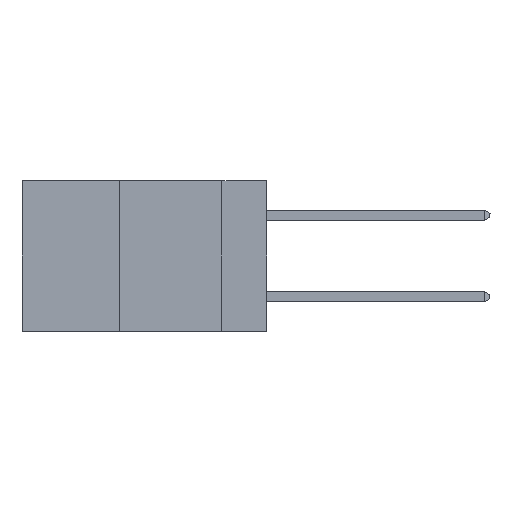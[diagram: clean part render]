
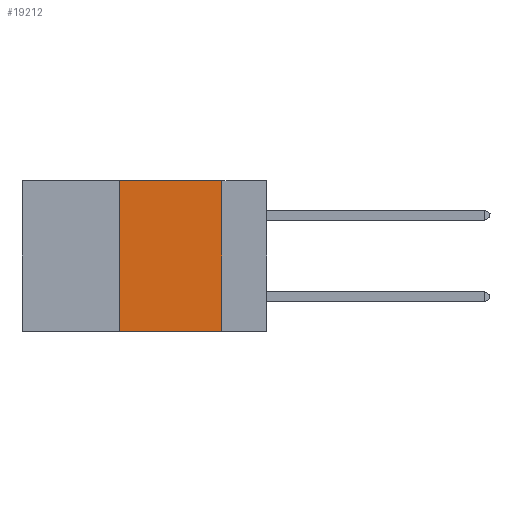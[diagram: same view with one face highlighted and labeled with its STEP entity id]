
A CAD part, left-side view. The second image highlights one B-rep face of the part: STEP entity #19212.
In plain terms, the highlighted planar face has unit normal (-1, 0, 0).
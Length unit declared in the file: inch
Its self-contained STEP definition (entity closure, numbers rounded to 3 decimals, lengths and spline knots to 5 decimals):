
#507 = VERTEX_POINT ( 'NONE', #23562 ) ;
#1046 = FACE_OUTER_BOUND ( 'NONE', #39341, .T. ) ;
#2009 = CARTESIAN_POINT ( 'NONE',  ( 0., 0.36, 0. ) ) ;
#2307 = CARTESIAN_POINT ( 'NONE',  ( 0., 0.36, -0.37 ) ) ;
#3094 = LINE ( 'NONE', #31910, #19514 ) ;
#3458 = DIRECTION ( 'NONE',  ( 0., -1., 0. ) ) ;
#4322 = ORIENTED_EDGE ( 'NONE', *, *, #38428, .T. ) ;
#7776 = DIRECTION ( 'NONE',  ( 1., 0., 0. ) ) ;
#9498 = DIRECTION ( 'NONE',  ( 0., -1., 0. ) ) ;
#9813 = DIRECTION ( 'NONE',  ( 0., 0., -1. ) ) ;
#10309 = VECTOR ( 'NONE', #3458, 39.37008 ) ;
#11929 = EDGE_CURVE ( 'NONE', #43889, #35983, #16713, .T. ) ;
#14010 = LINE ( 'NONE', #42127, #24287 ) ;
#14371 = CARTESIAN_POINT ( 'NONE',  ( 0., 0.6, -0.37 ) ) ;
#14750 = ORIENTED_EDGE ( 'NONE', *, *, #14943, .F. ) ;
#14763 = PLANE ( 'NONE',  #27522 ) ;
#14943 = EDGE_CURVE ( 'NONE', #35529, #43889, #3094, .T. ) ;
#16202 = CARTESIAN_POINT ( 'NONE',  ( 0., 0.11, 0. ) ) ;
#16713 = LINE ( 'NONE', #26956, #22000 ) ;
#19212 = ADVANCED_FACE ( 'NONE', ( #1046 ), #14763, .F. ) ;
#19514 = VECTOR ( 'NONE', #45849, 39.37008 ) ;
#22000 = VECTOR ( 'NONE', #9498, 39.37008 ) ;
#22433 = CARTESIAN_POINT ( 'NONE',  ( 0., 0.6, 0. ) ) ;
#22703 = ORIENTED_EDGE ( 'NONE', *, *, #45192, .F. ) ;
#23562 = CARTESIAN_POINT ( 'NONE',  ( 0., 0.11, -0.37 ) ) ;
#24287 = VECTOR ( 'NONE', #9813, 39.37008 ) ;
#26956 = CARTESIAN_POINT ( 'NONE',  ( 0., 0.6, 0. ) ) ;
#27522 = AXIS2_PLACEMENT_3D ( 'NONE', #22433, #7776, #36586 ) ;
#31910 = CARTESIAN_POINT ( 'NONE',  ( 0., 0.36, 0. ) ) ;
#35529 = VERTEX_POINT ( 'NONE', #2307 ) ;
#35983 = VERTEX_POINT ( 'NONE', #16202 ) ;
#36586 = DIRECTION ( 'NONE',  ( 0., 0., -1. ) ) ;
#38050 = ORIENTED_EDGE ( 'NONE', *, *, #11929, .F. ) ;
#38428 = EDGE_CURVE ( 'NONE', #35529, #507, #42964, .T. ) ;
#39341 = EDGE_LOOP ( 'NONE', ( #22703, #38050, #14750, #4322 ) ) ;
#42127 = CARTESIAN_POINT ( 'NONE',  ( 0., 0.11, 0. ) ) ;
#42964 = LINE ( 'NONE', #14371, #10309 ) ;
#43889 = VERTEX_POINT ( 'NONE', #2009 ) ;
#45192 = EDGE_CURVE ( 'NONE', #35983, #507, #14010, .T. ) ;
#45849 = DIRECTION ( 'NONE',  ( 0., 0., 1. ) ) ;
